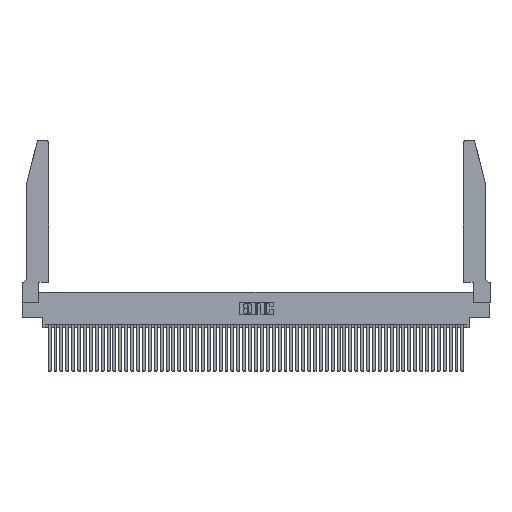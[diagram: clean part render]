
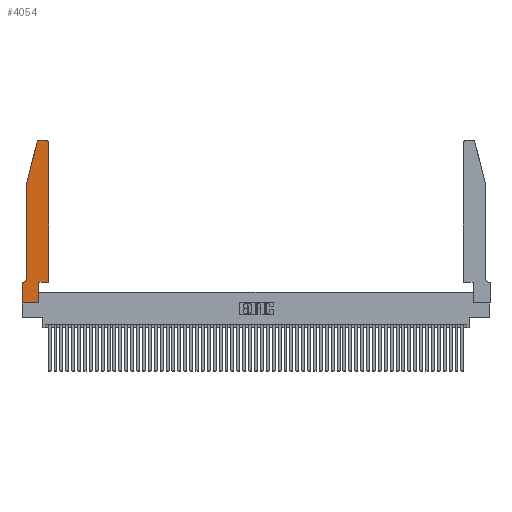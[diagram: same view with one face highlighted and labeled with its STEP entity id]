
A CAD part, top view. The second image highlights one B-rep face of the part: STEP entity #4054.
In plain terms, the highlighted planar face has unit normal (0, 0, 1).
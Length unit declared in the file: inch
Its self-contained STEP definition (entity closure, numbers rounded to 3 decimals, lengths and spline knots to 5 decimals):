
#2276 = CARTESIAN_POINT ( 'NONE',  ( 0.4505, 0.35, 0.37 ) ) ;
#2984 = ORIENTED_EDGE ( 'NONE', *, *, #13168, .T. ) ;
#3083 = ORIENTED_EDGE ( 'NONE', *, *, #33049, .T. ) ;
#3486 = VECTOR ( 'NONE', #54310, 39.37008 ) ;
#3582 = CARTESIAN_POINT ( 'NONE',  ( 0.0755, 0.35, 0.37 ) ) ;
#4054 = ADVANCED_FACE ( 'NONE', ( #14976 ), #24205, .T. ) ;
#4616 = VECTOR ( 'NONE', #41620, 39.37008 ) ;
#6759 = DIRECTION ( 'NONE',  ( 0., 0., 1. ) ) ;
#6969 = DIRECTION ( 'NONE',  ( 0., -1., 0. ) ) ;
#8442 = VERTEX_POINT ( 'NONE', #42603 ) ;
#8766 = EDGE_CURVE ( 'NONE', #51474, #35026, #18644, .T. ) ;
#8837 = AXIS2_PLACEMENT_3D ( 'NONE', #17841, #48330, #22273 ) ;
#8990 = VERTEX_POINT ( 'NONE', #15837 ) ;
#9119 = VECTOR ( 'NONE', #43470, 39.37008 ) ;
#10006 = CARTESIAN_POINT ( 'NONE',  ( 0.4205, 2.72, 0.37 ) ) ;
#10059 = VERTEX_POINT ( 'NONE', #34204 ) ;
#10111 = ORIENTED_EDGE ( 'NONE', *, *, #41981, .T. ) ;
#11496 = DIRECTION ( 'NONE',  ( 0., -1., 0. ) ) ;
#11797 = LINE ( 'NONE', #37480, #23469 ) ;
#12484 = ORIENTED_EDGE ( 'NONE', *, *, #45101, .T. ) ;
#13168 = EDGE_CURVE ( 'NONE', #48801, #22436, #39463, .T. ) ;
#14153 = CARTESIAN_POINT ( 'NONE',  ( 0.0055, 0.35, 0.37 ) ) ;
#14387 = DIRECTION ( 'NONE',  ( 1., 0., 0. ) ) ;
#14976 = FACE_OUTER_BOUND ( 'NONE', #29473, .T. ) ;
#15404 = ORIENTED_EDGE ( 'NONE', *, *, #39441, .T. ) ;
#15801 = AXIS2_PLACEMENT_3D ( 'NONE', #49358, #23341, #53749 ) ;
#15837 = CARTESIAN_POINT ( 'NONE',  ( 0.25487, 2.72718, 0.37 ) ) ;
#16545 = VECTOR ( 'NONE', #49989, 39.37008 ) ;
#17365 = ORIENTED_EDGE ( 'NONE', *, *, #18885, .T. ) ;
#17841 = CARTESIAN_POINT ( 'NONE',  ( 0.284, 2.72, 0.37 ) ) ;
#18233 = AXIS2_PLACEMENT_3D ( 'NONE', #32939, #6759, #37286 ) ;
#18580 = VERTEX_POINT ( 'NONE', #52361 ) ;
#18644 = CIRCLE ( 'NONE', #15801, 0.07 ) ;
#18885 = EDGE_CURVE ( 'NONE', #36372, #8442, #11797, .T. ) ;
#21615 = EDGE_CURVE ( 'NONE', #18580, #25547, #39557, .T. ) ;
#22273 = DIRECTION ( 'NONE',  ( 1., 0., 0. ) ) ;
#22436 = VERTEX_POINT ( 'NONE', #41231 ) ;
#23017 = AXIS2_PLACEMENT_3D ( 'NONE', #10006, #40531, #14387 ) ;
#23341 = DIRECTION ( 'NONE',  ( 0., 0., -1. ) ) ;
#23469 = VECTOR ( 'NONE', #6969, 39.37008 ) ;
#23684 = ORIENTED_EDGE ( 'NONE', *, *, #38530, .T. ) ;
#24205 = PLANE ( 'NONE',  #18233 ) ;
#24785 = ORIENTED_EDGE ( 'NONE', *, *, #8766, .T. ) ;
#24918 = DIRECTION ( 'NONE',  ( -1., 0., 0. ) ) ;
#25547 = VERTEX_POINT ( 'NONE', #51402 ) ;
#25855 = VECTOR ( 'NONE', #38536, 39.37008 ) ;
#28132 = VECTOR ( 'NONE', #11496, 39.37008 ) ;
#28149 = LINE ( 'NONE', #32636, #3486 ) ;
#28219 = EDGE_CURVE ( 'NONE', #8442, #45172, #48334, .T. ) ;
#29279 = CARTESIAN_POINT ( 'NONE',  ( 0.2605, 2.75, 0.37 ) ) ;
#29473 = EDGE_LOOP ( 'NONE', ( #35237, #56002, #15404, #3083, #24785, #12484, #17365, #38466, #10111, #2984, #23684, #44490 ) ) ;
#29543 = CARTESIAN_POINT ( 'NONE',  ( 0.2865, 0., 0.37 ) ) ;
#29938 = CARTESIAN_POINT ( 'NONE',  ( 0., 0., 0.37 ) ) ;
#30917 = VECTOR ( 'NONE', #24918, 39.37008 ) ;
#32308 = LINE ( 'NONE', #29279, #30917 ) ;
#32636 = CARTESIAN_POINT ( 'NONE',  ( 0.2865, 0.35, 0.37 ) ) ;
#32939 = CARTESIAN_POINT ( 'NONE',  ( 0., 0.35, 0.37 ) ) ;
#33049 = EDGE_CURVE ( 'NONE', #49773, #51474, #51270, .T. ) ;
#33317 = CARTESIAN_POINT ( 'NONE',  ( 0.0755, 2., 0.37 ) ) ;
#33603 = CARTESIAN_POINT ( 'NONE',  ( 0., 0.35, 0.37 ) ) ;
#34204 = CARTESIAN_POINT ( 'NONE',  ( 0.284, 2.75, 0.37 ) ) ;
#35026 = VERTEX_POINT ( 'NONE', #14153 ) ;
#35027 = CIRCLE ( 'NONE', #8837, 0.03 ) ;
#35237 = ORIENTED_EDGE ( 'NONE', *, *, #41420, .T. ) ;
#36372 = VERTEX_POINT ( 'NONE', #33603 ) ;
#36852 = CARTESIAN_POINT ( 'NONE',  ( 0.0755, 2., 0.37 ) ) ;
#37286 = DIRECTION ( 'NONE',  ( 1., 0., 0. ) ) ;
#37365 = LINE ( 'NONE', #3582, #25855 ) ;
#37480 = CARTESIAN_POINT ( 'NONE',  ( 0., 0., 0.37 ) ) ;
#38466 = ORIENTED_EDGE ( 'NONE', *, *, #28219, .T. ) ;
#38530 = EDGE_CURVE ( 'NONE', #22436, #18580, #55525, .T. ) ;
#38536 = DIRECTION ( 'NONE',  ( -1., 0., 0. ) ) ;
#39441 = EDGE_CURVE ( 'NONE', #8990, #49773, #41108, .T. ) ;
#39463 = LINE ( 'NONE', #2276, #4616 ) ;
#39557 = CIRCLE ( 'NONE', #23017, 0.03 ) ;
#40531 = DIRECTION ( 'NONE',  ( 0., 0., 1. ) ) ;
#41108 = LINE ( 'NONE', #36852, #16545 ) ;
#41231 = CARTESIAN_POINT ( 'NONE',  ( 0.4505, 0.35, 0.37 ) ) ;
#41420 = EDGE_CURVE ( 'NONE', #25547, #10059, #32308, .T. ) ;
#41469 = CARTESIAN_POINT ( 'NONE',  ( 0.0755, 2., 0.37 ) ) ;
#41620 = DIRECTION ( 'NONE',  ( 1., 0., 0. ) ) ;
#41981 = EDGE_CURVE ( 'NONE', #45172, #48801, #28149, .T. ) ;
#42603 = CARTESIAN_POINT ( 'NONE',  ( 0., 0., 0.37 ) ) ;
#43470 = DIRECTION ( 'NONE',  ( 0., 1., 0. ) ) ;
#44490 = ORIENTED_EDGE ( 'NONE', *, *, #21615, .T. ) ;
#45101 = EDGE_CURVE ( 'NONE', #35026, #36372, #37365, .T. ) ;
#45172 = VERTEX_POINT ( 'NONE', #29543 ) ;
#46974 = VECTOR ( 'NONE', #51606, 39.37008 ) ;
#47658 = CARTESIAN_POINT ( 'NONE',  ( 0.4505, 0.35, 0.37 ) ) ;
#48037 = CARTESIAN_POINT ( 'NONE',  ( 0.2865, 0.35, 0.37 ) ) ;
#48330 = DIRECTION ( 'NONE',  ( 0., 0., 1. ) ) ;
#48334 = LINE ( 'NONE', #29938, #46974 ) ;
#48801 = VERTEX_POINT ( 'NONE', #48037 ) ;
#49358 = CARTESIAN_POINT ( 'NONE',  ( 0.0055, 0.42, 0.37 ) ) ;
#49492 = EDGE_CURVE ( 'NONE', #10059, #8990, #35027, .T. ) ;
#49773 = VERTEX_POINT ( 'NONE', #41469 ) ;
#49989 = DIRECTION ( 'NONE',  ( -0.239, -0.971, 0. ) ) ;
#51270 = LINE ( 'NONE', #33317, #28132 ) ;
#51402 = CARTESIAN_POINT ( 'NONE',  ( 0.4205, 2.75, 0.37 ) ) ;
#51474 = VERTEX_POINT ( 'NONE', #52824 ) ;
#51606 = DIRECTION ( 'NONE',  ( 1., 0., 0. ) ) ;
#52361 = CARTESIAN_POINT ( 'NONE',  ( 0.4505, 2.72, 0.37 ) ) ;
#52824 = CARTESIAN_POINT ( 'NONE',  ( 0.0755, 0.42, 0.37 ) ) ;
#53749 = DIRECTION ( 'NONE',  ( -1., 0., 0. ) ) ;
#54310 = DIRECTION ( 'NONE',  ( 0., 1., 0. ) ) ;
#55525 = LINE ( 'NONE', #47658, #9119 ) ;
#56002 = ORIENTED_EDGE ( 'NONE', *, *, #49492, .T. ) ;
